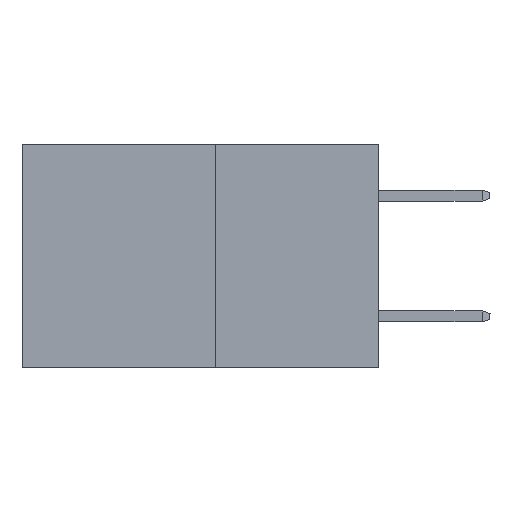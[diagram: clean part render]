
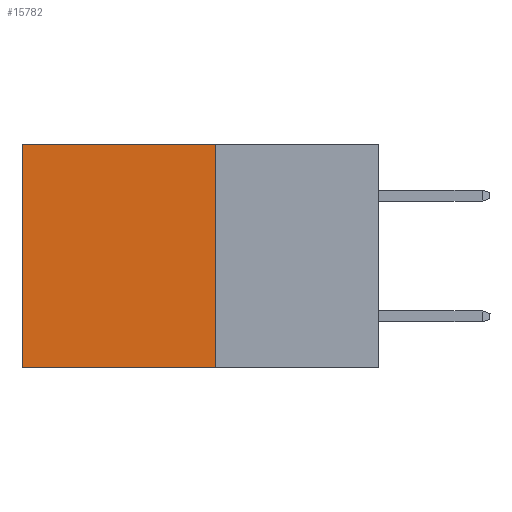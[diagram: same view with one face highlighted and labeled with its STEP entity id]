
A CAD part, left-side view. The second image highlights one B-rep face of the part: STEP entity #15782.
In plain terms, the highlighted planar face has unit normal (-1, 0, 0).
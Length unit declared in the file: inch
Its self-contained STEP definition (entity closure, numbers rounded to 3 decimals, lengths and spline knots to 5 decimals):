
#569 = VECTOR ( 'NONE', #3647, 39.37008 ) ;
#805 = DIRECTION ( 'NONE',  ( 1., 0., 0. ) ) ;
#1341 = LINE ( 'NONE', #20502, #569 ) ;
#2323 = CARTESIAN_POINT ( 'NONE',  ( 0.277, 0.59, 0. ) ) ;
#2921 = CARTESIAN_POINT ( 'NONE',  ( 0.277, 0.27, 0. ) ) ;
#3647 = DIRECTION ( 'NONE',  ( 0., 0., -1. ) ) ;
#4839 = AXIS2_PLACEMENT_3D ( 'NONE', #14534, #805, #16924 ) ;
#5055 = EDGE_LOOP ( 'NONE', ( #27031, #28467, #19265, #11879 ) ) ;
#5687 = DIRECTION ( 'NONE',  ( 0., 1., 0. ) ) ;
#6840 = LINE ( 'NONE', #24899, #25239 ) ;
#7341 = VECTOR ( 'NONE', #22187, 39.37008 ) ;
#8788 = EDGE_CURVE ( 'NONE', #20927, #21287, #1341, .T. ) ;
#9194 = CARTESIAN_POINT ( 'NONE',  ( 0.277, 0.27, -0.37 ) ) ;
#10623 = EDGE_CURVE ( 'NONE', #11283, #20927, #25712, .T. ) ;
#11283 = VERTEX_POINT ( 'NONE', #19752 ) ;
#11879 = ORIENTED_EDGE ( 'NONE', *, *, #10623, .T. ) ;
#13308 = FACE_OUTER_BOUND ( 'NONE', #5055, .T. ) ;
#13935 = LINE ( 'NONE', #21291, #19519 ) ;
#14435 = PLANE ( 'NONE',  #4839 ) ;
#14534 = CARTESIAN_POINT ( 'NONE',  ( 0.277, 0.27, -0.37 ) ) ;
#15003 = VERTEX_POINT ( 'NONE', #9194 ) ;
#15782 = ADVANCED_FACE ( 'NONE', ( #13308 ), #14435, .F. ) ;
#16924 = DIRECTION ( 'NONE',  ( 0., 0., -1. ) ) ;
#19265 = ORIENTED_EDGE ( 'NONE', *, *, #20854, .F. ) ;
#19519 = VECTOR ( 'NONE', #30876, 39.37008 ) ;
#19752 = CARTESIAN_POINT ( 'NONE',  ( 0.277, 0.27, 0. ) ) ;
#20502 = CARTESIAN_POINT ( 'NONE',  ( 0.277, 0.59, -0.37 ) ) ;
#20854 = EDGE_CURVE ( 'NONE', #11283, #15003, #13935, .T. ) ;
#20927 = VERTEX_POINT ( 'NONE', #2323 ) ;
#21287 = VERTEX_POINT ( 'NONE', #21523 ) ;
#21291 = CARTESIAN_POINT ( 'NONE',  ( 0.277, 0.27, -0.37 ) ) ;
#21523 = CARTESIAN_POINT ( 'NONE',  ( 0.277, 0.59, -0.37 ) ) ;
#22187 = DIRECTION ( 'NONE',  ( 0., 1., 0. ) ) ;
#24899 = CARTESIAN_POINT ( 'NONE',  ( 0.277, 0.27, -0.37 ) ) ;
#25239 = VECTOR ( 'NONE', #5687, 39.37008 ) ;
#25712 = LINE ( 'NONE', #2921, #7341 ) ;
#27031 = ORIENTED_EDGE ( 'NONE', *, *, #8788, .T. ) ;
#27314 = EDGE_CURVE ( 'NONE', #15003, #21287, #6840, .T. ) ;
#28467 = ORIENTED_EDGE ( 'NONE', *, *, #27314, .F. ) ;
#30876 = DIRECTION ( 'NONE',  ( 0., 0., -1. ) ) ;
